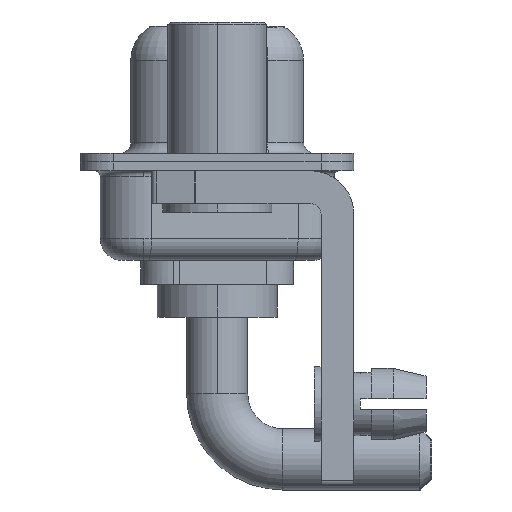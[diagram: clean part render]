
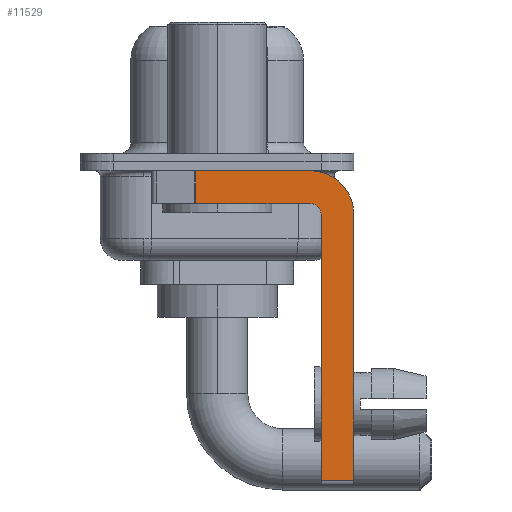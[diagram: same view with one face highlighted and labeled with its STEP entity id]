
A CAD part, left-side view. The second image highlights one B-rep face of the part: STEP entity #11529.
In plain terms, the highlighted planar face has unit normal (-1, 0, 0).
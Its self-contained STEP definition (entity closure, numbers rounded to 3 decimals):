
#178 = CARTESIAN_POINT ( 'NONE',  ( -2.9, -6.25, -14.55 ) ) ;
#311 = CARTESIAN_POINT ( 'NONE',  ( -2.9, -4.75, -2.4 ) ) ;
#339 = VERTEX_POINT ( 'NONE', #11831 ) ;
#368 = VERTEX_POINT ( 'NONE', #14535 ) ;
#523 = CARTESIAN_POINT ( 'NONE',  ( -2.9, -6.25, -2.4 ) ) ;
#548 = EDGE_LOOP ( 'NONE', ( #5225, #2372, #7394, #1255, #675, #7706, #16795, #3179 ) ) ;
#675 = ORIENTED_EDGE ( 'NONE', *, *, #2375, .F. ) ;
#687 = FACE_OUTER_BOUND ( 'NONE', #548, .T. ) ;
#716 = CARTESIAN_POINT ( 'NONE',  ( -2.9, -4.75, -14.8 ) ) ;
#805 = CARTESIAN_POINT ( 'NONE',  ( -2.9, -4.25, -2.4 ) ) ;
#883 = DIRECTION ( 'NONE',  ( 0., 1., 0. ) ) ;
#970 = CARTESIAN_POINT ( 'NONE',  ( -2.9, -4.25, -14.55 ) ) ;
#1061 = DIRECTION ( 'NONE',  ( 0., 0., -1. ) ) ;
#1156 = VERTEX_POINT ( 'NONE', #8768 ) ;
#1255 = ORIENTED_EDGE ( 'NONE', *, *, #1909, .F. ) ;
#1884 = EDGE_CURVE ( 'NONE', #13397, #368, #17214, .T. ) ;
#1909 = EDGE_CURVE ( 'NONE', #6331, #339, #13709, .T. ) ;
#2070 = CARTESIAN_POINT ( 'NONE',  ( -2.9, 3., -0.4 ) ) ;
#2097 = DIRECTION ( 'NONE',  ( 1., 0., 0. ) ) ;
#2147 = DIRECTION ( 'NONE',  ( -1., 0., 0. ) ) ;
#2219 = EDGE_CURVE ( 'NONE', #7657, #11288, #9562, .T. ) ;
#2372 = ORIENTED_EDGE ( 'NONE', *, *, #1884, .T. ) ;
#2375 = EDGE_CURVE ( 'NONE', #1156, #6331, #17015, .T. ) ;
#2688 = LINE ( 'NONE', #523, #11961 ) ;
#3039 = CARTESIAN_POINT ( 'NONE',  ( -2.9, 0.978, -0.4 ) ) ;
#3179 = ORIENTED_EDGE ( 'NONE', *, *, #2219, .F. ) ;
#3436 = LINE ( 'NONE', #970, #13286 ) ;
#3648 = DIRECTION ( 'NONE',  ( 0., -1., 0. ) ) ;
#3678 = VECTOR ( 'NONE', #14469, 1000. ) ;
#4233 = AXIS2_PLACEMENT_3D ( 'NONE', #805, #16756, #1061 ) ;
#4669 = EDGE_CURVE ( 'NONE', #13397, #7657, #12832, .T. ) ;
#4731 = DIRECTION ( 'NONE',  ( 0., 0., -1. ) ) ;
#5225 = ORIENTED_EDGE ( 'NONE', *, *, #4669, .F. ) ;
#5532 = EDGE_CURVE ( 'NONE', #339, #368, #15511, .T. ) ;
#6055 = CARTESIAN_POINT ( 'NONE',  ( -2.9, -4.25, -2.4 ) ) ;
#6331 = VERTEX_POINT ( 'NONE', #311 ) ;
#7394 = ORIENTED_EDGE ( 'NONE', *, *, #5532, .F. ) ;
#7398 = VECTOR ( 'NONE', #3648, 1000. ) ;
#7494 = DIRECTION ( 'NONE',  ( 0., 0., 1. ) ) ;
#7657 = VERTEX_POINT ( 'NONE', #14912 ) ;
#7706 = ORIENTED_EDGE ( 'NONE', *, *, #7942, .T. ) ;
#7942 = EDGE_CURVE ( 'NONE', #1156, #8081, #3436, .T. ) ;
#8081 = VERTEX_POINT ( 'NONE', #178 ) ;
#8768 = CARTESIAN_POINT ( 'NONE',  ( -2.9, -4.75, -14.55 ) ) ;
#9007 = CARTESIAN_POINT ( 'NONE',  ( -2.9, -4.25, -2.4 ) ) ;
#9549 = VECTOR ( 'NONE', #10305, 1000. ) ;
#9562 = CIRCLE ( 'NONE', #4233, 2. ) ;
#10305 = DIRECTION ( 'NONE',  ( 0., 0., -1. ) ) ;
#10400 = CARTESIAN_POINT ( 'NONE',  ( -2.9, 0.978, -1.9 ) ) ;
#11288 = VERTEX_POINT ( 'NONE', #14115 ) ;
#11492 = AXIS2_PLACEMENT_3D ( 'NONE', #9007, #2147, #7494 ) ;
#11497 = CARTESIAN_POINT ( 'NONE',  ( -2.9, -4.25, -1.9 ) ) ;
#11529 = ADVANCED_FACE ( 'NONE', ( #687 ), #13909, .F. ) ;
#11831 = CARTESIAN_POINT ( 'NONE',  ( -2.9, -4.25, -1.9 ) ) ;
#11961 = VECTOR ( 'NONE', #14663, 1000. ) ;
#12796 = DIRECTION ( 'NONE',  ( 0., -1., 0. ) ) ;
#12832 = LINE ( 'NONE', #2070, #7398 ) ;
#13052 = AXIS2_PLACEMENT_3D ( 'NONE', #6055, #2097, #4731 ) ;
#13286 = VECTOR ( 'NONE', #12796, 1000. ) ;
#13397 = VERTEX_POINT ( 'NONE', #3039 ) ;
#13709 = CIRCLE ( 'NONE', #11492, 0.5 ) ;
#13909 = PLANE ( 'NONE',  #13052 ) ;
#13925 = EDGE_CURVE ( 'NONE', #11288, #8081, #2688, .T. ) ;
#14115 = CARTESIAN_POINT ( 'NONE',  ( -2.9, -6.25, -2.4 ) ) ;
#14469 = DIRECTION ( 'NONE',  ( 0., 0., 1. ) ) ;
#14535 = CARTESIAN_POINT ( 'NONE',  ( -2.9, 0.978, -1.9 ) ) ;
#14663 = DIRECTION ( 'NONE',  ( 0., 0., -1. ) ) ;
#14912 = CARTESIAN_POINT ( 'NONE',  ( -2.9, -4.25, -0.4 ) ) ;
#15511 = LINE ( 'NONE', #11497, #15811 ) ;
#15811 = VECTOR ( 'NONE', #883, 1000. ) ;
#16756 = DIRECTION ( 'NONE',  ( 1., 0., 0. ) ) ;
#16795 = ORIENTED_EDGE ( 'NONE', *, *, #13925, .F. ) ;
#17015 = LINE ( 'NONE', #716, #3678 ) ;
#17214 = LINE ( 'NONE', #10400, #9549 ) ;
